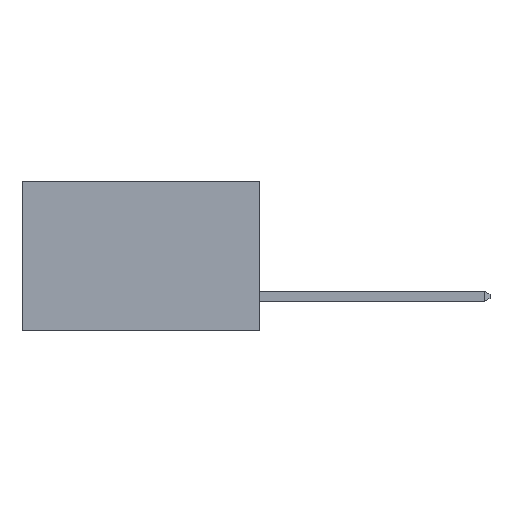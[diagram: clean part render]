
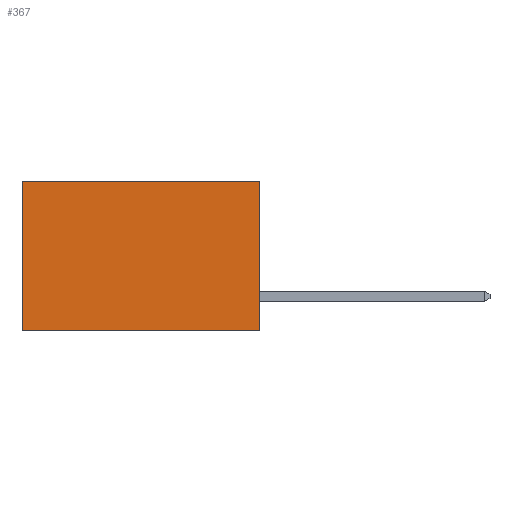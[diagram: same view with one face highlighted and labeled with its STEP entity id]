
A CAD part, left-side view. The second image highlights one B-rep face of the part: STEP entity #367.
In plain terms, the highlighted planar face has unit normal (-1, 0, 0).
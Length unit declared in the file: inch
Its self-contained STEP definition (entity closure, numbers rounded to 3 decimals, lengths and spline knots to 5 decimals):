
#132 = DIRECTION ( 'NONE',  ( 0., 1., 0. ) ) ;
#211 = CARTESIAN_POINT ( 'NONE',  ( 0.277, 0., 0. ) ) ;
#259 = CARTESIAN_POINT ( 'NONE',  ( 0.277, 0.59, -0.37 ) ) ;
#367 = ADVANCED_FACE ( 'NONE', ( #5712 ), #8413, .F. ) ;
#1065 = VERTEX_POINT ( 'NONE', #8319 ) ;
#2254 = LINE ( 'NONE', #211, #5559 ) ;
#2432 = AXIS2_PLACEMENT_3D ( 'NONE', #5099, #8281, #8261 ) ;
#2560 = VECTOR ( 'NONE', #5097, 39.37008 ) ;
#2989 = LINE ( 'NONE', #4811, #7974 ) ;
#3508 = EDGE_CURVE ( 'NONE', #7082, #1065, #2989, .T. ) ;
#3943 = VECTOR ( 'NONE', #5630, 39.37008 ) ;
#4136 = CARTESIAN_POINT ( 'NONE',  ( 0.277, 0.59, -0.37 ) ) ;
#4300 = ORIENTED_EDGE ( 'NONE', *, *, #5165, .T. ) ;
#4336 = LINE ( 'NONE', #5090, #2560 ) ;
#4510 = ORIENTED_EDGE ( 'NONE', *, *, #3508, .F. ) ;
#4553 = ORIENTED_EDGE ( 'NONE', *, *, #5342, .F. ) ;
#4591 = ORIENTED_EDGE ( 'NONE', *, *, #4930, .T. ) ;
#4596 = EDGE_LOOP ( 'NONE', ( #4591, #4553, #4510, #4300 ) ) ;
#4633 = VERTEX_POINT ( 'NONE', #6770 ) ;
#4644 = DIRECTION ( 'NONE',  ( 0., 0., -1. ) ) ;
#4811 = CARTESIAN_POINT ( 'NONE',  ( 0.277, 0., -0.37 ) ) ;
#4930 = EDGE_CURVE ( 'NONE', #4633, #6650, #7378, .T. ) ;
#5090 = CARTESIAN_POINT ( 'NONE',  ( 0.277, 0., -0.37 ) ) ;
#5097 = DIRECTION ( 'NONE',  ( 0., 1., 0. ) ) ;
#5099 = CARTESIAN_POINT ( 'NONE',  ( 0.277, 0., -0.37 ) ) ;
#5165 = EDGE_CURVE ( 'NONE', #7082, #4633, #2254, .T. ) ;
#5342 = EDGE_CURVE ( 'NONE', #1065, #6650, #4336, .T. ) ;
#5559 = VECTOR ( 'NONE', #132, 39.37008 ) ;
#5630 = DIRECTION ( 'NONE',  ( 0., 0., -1. ) ) ;
#5712 = FACE_OUTER_BOUND ( 'NONE', #4596, .T. ) ;
#6650 = VERTEX_POINT ( 'NONE', #4136 ) ;
#6770 = CARTESIAN_POINT ( 'NONE',  ( 0.277, 0.59, 0. ) ) ;
#7082 = VERTEX_POINT ( 'NONE', #7225 ) ;
#7225 = CARTESIAN_POINT ( 'NONE',  ( 0.277, 0., 0. ) ) ;
#7378 = LINE ( 'NONE', #259, #3943 ) ;
#7974 = VECTOR ( 'NONE', #4644, 39.37008 ) ;
#8261 = DIRECTION ( 'NONE',  ( 0., 0., -1. ) ) ;
#8281 = DIRECTION ( 'NONE',  ( 1., 0., 0. ) ) ;
#8319 = CARTESIAN_POINT ( 'NONE',  ( 0.277, 0., -0.37 ) ) ;
#8413 = PLANE ( 'NONE',  #2432 ) ;
